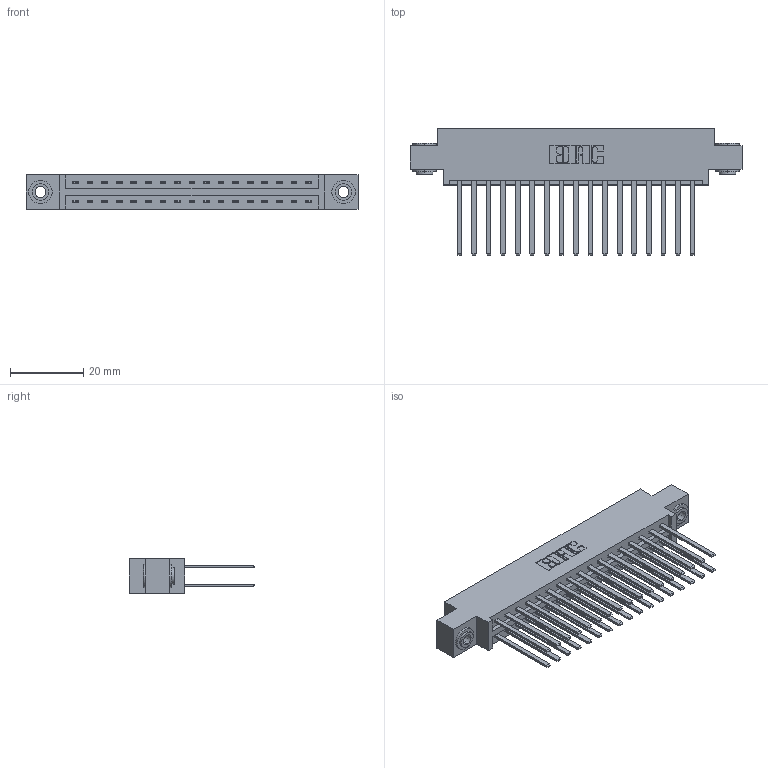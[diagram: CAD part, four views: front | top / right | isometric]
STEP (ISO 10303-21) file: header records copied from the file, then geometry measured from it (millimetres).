
FILE_DESCRIPTION (( 'STEP AP203' ), '1' );
FILE_NAME ('337-034-544-803.STEP', '2018-08-07T12:59:56', ( '' ), ( '' ), 'SwSTEP 2.0', 'SolidWorks 2016', '' );
FILE_SCHEMA (( 'CONFIG_CONTROL_DESIGN' ));
Length unit declared in the file: inch
Products named in the file (4): 337 Part_0.170 Offset - 0.156 Dia-TH; 345-292-001_345-293-144; 345-250-002_345-250-002-102; 337-034-544-803
Assembly tree (37 placements, depth 2):
  337-034-544-803
    337 Part_0.170 Offset - 0.156 Dia-TH
    345-292-001_345-293-144  x34
    345-250-002_345-250-002-102  x2
Bounding box: 90.37 x 34.3 x 9.4 mm (x, y, z)
Volume: 9570 mm3; surface area: 12465.3 mm2
Topology: 37 solids, 37 shells, 1788 faces, 5261 edges, 3458 vertices
Faces by surface type: plane 1240, cylinder 540, cone 8
Entity records: 17012 total; most frequent: CARTESIAN_POINT 2861, ORIENTED_EDGE 2790, DIRECTION 2509, EDGE_CURVE 1395, LINE 1247, VECTOR 1247, VERTEX_POINT 926, AXIS2_PLACEMENT_3D 631
